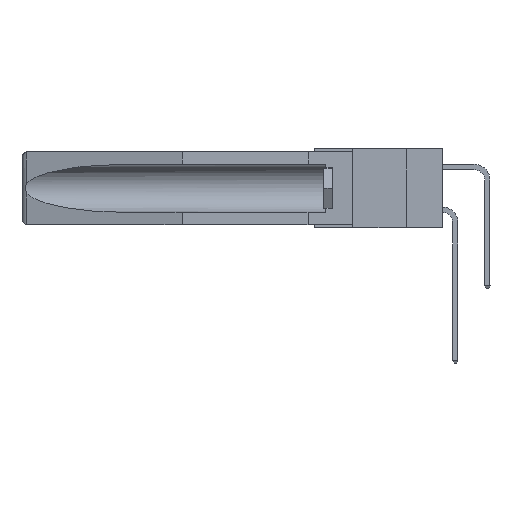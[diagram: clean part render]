
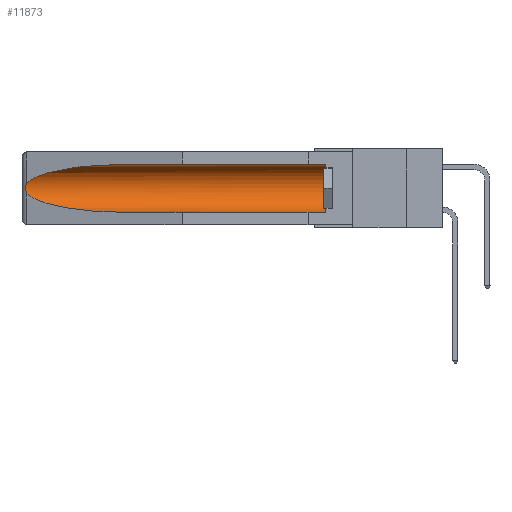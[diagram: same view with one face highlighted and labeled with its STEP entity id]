
A CAD part, left-side view. The second image highlights one B-rep face of the part: STEP entity #11873.
In plain terms, the highlighted cylindrical face has radius 2.857 mm (diameter 5.715 mm), a partial arc.
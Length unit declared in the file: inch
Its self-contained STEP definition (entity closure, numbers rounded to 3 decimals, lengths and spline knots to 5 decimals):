
#354 = AXIS2_PLACEMENT_3D ( 'NONE', #15217, #11016, #8100 ) ;
#365 = VERTEX_POINT ( 'NONE', #12104 ) ;
#657 = CARTESIAN_POINT ( 'NONE',  ( 0.26537, 1.52718, -0.14972 ) ) ;
#718 = CARTESIAN_POINT ( 'NONE',  ( 0.26537, 1.52718, -0.19328 ) ) ;
#939 = VERTEX_POINT ( 'NONE', #12065 ) ;
#1312 = EDGE_CURVE ( 'NONE', #365, #3949, #10577, .T. ) ;
#1533 = DIRECTION ( 'NONE',  ( 0., 1., 0. ) ) ;
#1929 = B_SPLINE_CURVE_WITH_KNOTS ( 'NONE', 3,
 ( #11112, #3813, #16887, #15498, #13669, #5431, #9346, #3931, #16949, #8378 ),
 .UNSPECIFIED., .F., .F.,
 ( 4, 2, 2, 2, 4 ),
 ( 0., 0.00029, 0.00058, 0.00087, 0.00117 ),
 .UNSPECIFIED. ) ;
#2004 = EDGE_CURVE ( 'NONE', #13375, #939, #13531, .T. ) ;
#2669 = EDGE_CURVE ( 'NONE', #13336, #13375, #1929, .T. ) ;
#2982 = EDGE_CURVE ( 'NONE', #365, #939, #9859, .T. ) ;
#3155 = ORIENTED_EDGE ( 'NONE', *, *, #1312, .T. ) ;
#3189 = EDGE_LOOP ( 'NONE', ( #18155, #8004, #9114, #6122, #3155, #14592 ) ) ;
#3813 = CARTESIAN_POINT ( 'NONE',  ( 0.26597, 1.52961, -0.15275 ) ) ;
#3838 = AXIS2_PLACEMENT_3D ( 'NONE', #8463, #14261, #15763 ) ;
#3931 = CARTESIAN_POINT ( 'NONE',  ( 0.26655, 1.53094, -0.18657 ) ) ;
#3949 = VERTEX_POINT ( 'NONE', #15491 ) ;
#4232 = CARTESIAN_POINT ( 'NONE',  ( 0.26537, 1.52718, -0.19328 ) ) ;
#4290 = CARTESIAN_POINT ( 'NONE',  ( 0.155, 1.07973, -0.284 ) ) ;
#4338 = VECTOR ( 'NONE', #1533, 39.37008 ) ;
#4409 = CARTESIAN_POINT ( 'NONE',  ( 0.155, 1.07973, -0.059 ) ) ;
#5431 = CARTESIAN_POINT ( 'NONE',  ( 0.2675, 1.53308, -0.17534 ) ) ;
#6122 = ORIENTED_EDGE ( 'NONE', *, *, #2982, .F. ) ;
#6242 = VERTEX_POINT ( 'NONE', #4409 ) ;
#6353 = CARTESIAN_POINT ( 'NONE',  ( 0.155, 1.07973, -0.059 ) ) ;
#8004 = ORIENTED_EDGE ( 'NONE', *, *, #2669, .T. ) ;
#8100 = DIRECTION ( 'NONE',  ( 0., 0., 1. ) ) ;
#8183 = VECTOR ( 'NONE', #12978, 39.37008 ) ;
#8378 = CARTESIAN_POINT ( 'NONE',  ( 0.26537, 1.52718, -0.19328 ) ) ;
#8463 = CARTESIAN_POINT ( 'NONE',  ( 0.155, -0.30754, -0.1715 ) ) ;
#9114 = ORIENTED_EDGE ( 'NONE', *, *, #2004, .T. ) ;
#9301 = CARTESIAN_POINT ( 'NONE',  ( 0.26537, 1.52718, -0.14972 ) ) ;
#9346 = CARTESIAN_POINT ( 'NONE',  ( 0.2673, 1.53269, -0.17917 ) ) ;
#9439 = EDGE_CURVE ( 'NONE', #6242, #13336, #12829, .T. ) ;
#9859 = LINE ( 'NONE', #11810, #4338 ) ;
#10577 = CIRCLE ( 'NONE', #354, 0.1125 ) ;
#10818 = CARTESIAN_POINT ( 'NONE',  ( 0.25451, 1.48313, -0.09465 ) ) ;
#11016 = DIRECTION ( 'NONE',  ( 0., -1., 0. ) ) ;
#11112 = CARTESIAN_POINT ( 'NONE',  ( 0.26537, 1.52718, -0.14972 ) ) ;
#11343 = EDGE_CURVE ( 'NONE', #3949, #6242, #11819, .T. ) ;
#11810 = CARTESIAN_POINT ( 'NONE',  ( 0.155, -0.30754, -0.284 ) ) ;
#11819 = LINE ( 'NONE', #15955, #8183 ) ;
#11873 = ADVANCED_FACE ( 'NONE', ( #13417 ), #14100, .F. ) ;
#12065 = CARTESIAN_POINT ( 'NONE',  ( 0.155, 1.07973, -0.284 ) ) ;
#12104 = CARTESIAN_POINT ( 'NONE',  ( 0.155, 0.126, -0.284 ) ) ;
#12164 = CARTESIAN_POINT ( 'NONE',  ( 0.21114, 1.30732, -0.059 ) ) ;
#12829 =( BOUNDED_CURVE ( )  B_SPLINE_CURVE ( 3, ( #6353, #12164, #10818, #657 ),
 .UNSPECIFIED., .F., .F. ) 
 B_SPLINE_CURVE_WITH_KNOTS ( ( 4, 4 ),
 ( 4.71239, 6.08839 ),
 .UNSPECIFIED. ) 
 CURVE ( )  GEOMETRIC_REPRESENTATION_ITEM ( )  RATIONAL_B_SPLINE_CURVE ( ( 1., 0.848, 0.848, 1. ) ) 
 REPRESENTATION_ITEM ( '' )  );
#12978 = DIRECTION ( 'NONE',  ( 0., 1., 0. ) ) ;
#13336 = VERTEX_POINT ( 'NONE', #9301 ) ;
#13375 = VERTEX_POINT ( 'NONE', #718 ) ;
#13417 = FACE_OUTER_BOUND ( 'NONE', #3189, .T. ) ;
#13531 =( BOUNDED_CURVE ( )  B_SPLINE_CURVE ( 3, ( #4232, #18754, #17360, #4290 ),
 .UNSPECIFIED., .F., .F. ) 
 B_SPLINE_CURVE_WITH_KNOTS ( ( 4, 4 ),
 ( 0.1948, 1.5708 ),
 .UNSPECIFIED. ) 
 CURVE ( )  GEOMETRIC_REPRESENTATION_ITEM ( )  RATIONAL_B_SPLINE_CURVE ( ( 1., 0.848, 0.848, 1. ) ) 
 REPRESENTATION_ITEM ( '' )  );
#13669 = CARTESIAN_POINT ( 'NONE',  ( 0.2675, 1.53308, -0.16763 ) ) ;
#14100 = CYLINDRICAL_SURFACE ( 'NONE', #3838, 0.1125 ) ;
#14261 = DIRECTION ( 'NONE',  ( 0., 1., 0. ) ) ;
#14592 = ORIENTED_EDGE ( 'NONE', *, *, #11343, .T. ) ;
#15217 = CARTESIAN_POINT ( 'NONE',  ( 0.155, 0.126, -0.1715 ) ) ;
#15491 = CARTESIAN_POINT ( 'NONE',  ( 0.155, 0.126, -0.059 ) ) ;
#15498 = CARTESIAN_POINT ( 'NONE',  ( 0.2673, 1.5327, -0.16383 ) ) ;
#15763 = DIRECTION ( 'NONE',  ( 0., 0., 1. ) ) ;
#15955 = CARTESIAN_POINT ( 'NONE',  ( 0.155, -0.30754, -0.059 ) ) ;
#16887 = CARTESIAN_POINT ( 'NONE',  ( 0.26654, 1.53092, -0.15636 ) ) ;
#16949 = CARTESIAN_POINT ( 'NONE',  ( 0.26597, 1.5296, -0.19026 ) ) ;
#17360 = CARTESIAN_POINT ( 'NONE',  ( 0.21114, 1.30732, -0.284 ) ) ;
#18155 = ORIENTED_EDGE ( 'NONE', *, *, #9439, .T. ) ;
#18754 = CARTESIAN_POINT ( 'NONE',  ( 0.25451, 1.48313, -0.24835 ) ) ;
